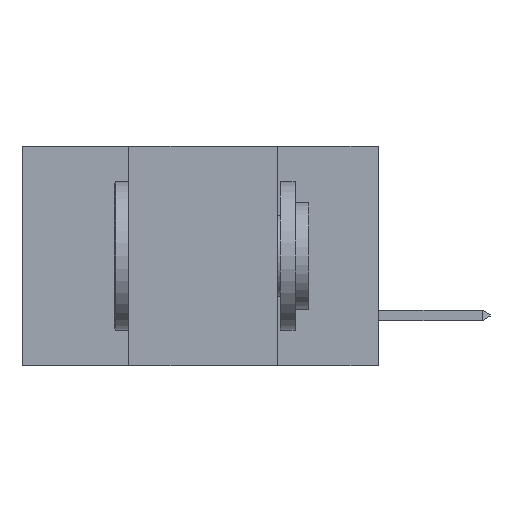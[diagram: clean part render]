
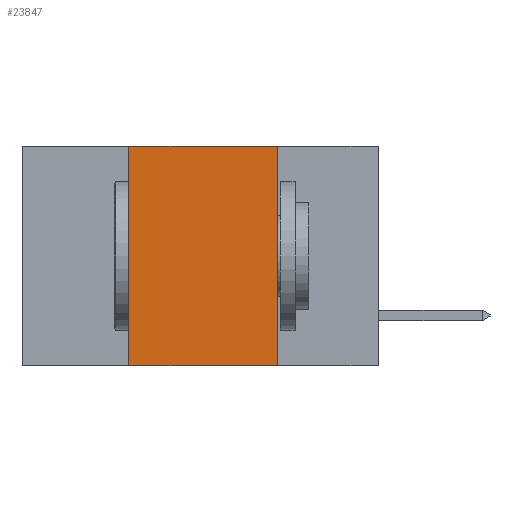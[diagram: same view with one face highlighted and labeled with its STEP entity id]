
A CAD part, left-side view. The second image highlights one B-rep face of the part: STEP entity #23847.
In plain terms, the highlighted planar face has unit normal (-1, 0, 0).
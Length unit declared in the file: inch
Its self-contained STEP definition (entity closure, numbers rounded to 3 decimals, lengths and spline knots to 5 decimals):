
#33 = VECTOR ( 'NONE', #9868, 39.37008 ) ;
#68 = LINE ( 'NONE', #454, #15232 ) ;
#454 = CARTESIAN_POINT ( 'NONE',  ( 0., 0.42, 0. ) ) ;
#1614 = CARTESIAN_POINT ( 'NONE',  ( 0., 0.42, 0. ) ) ;
#2110 = EDGE_CURVE ( 'NONE', #12741, #16547, #10633, .T. ) ;
#2787 = EDGE_CURVE ( 'NONE', #6114, #9999, #25137, .T. ) ;
#3353 = CARTESIAN_POINT ( 'NONE',  ( 0., 0.6, -0.37 ) ) ;
#3735 = ORIENTED_EDGE ( 'NONE', *, *, #16699, .F. ) ;
#4268 = CARTESIAN_POINT ( 'NONE',  ( 0., 0.17, -0.37 ) ) ;
#5247 = EDGE_LOOP ( 'NONE', ( #3735, #24932, #14243, #9458 ) ) ;
#5860 = PLANE ( 'NONE',  #14925 ) ;
#6114 = VERTEX_POINT ( 'NONE', #1614 ) ;
#9458 = ORIENTED_EDGE ( 'NONE', *, *, #2110, .T. ) ;
#9756 = DIRECTION ( 'NONE',  ( 0., 0., -1. ) ) ;
#9868 = DIRECTION ( 'NONE',  ( 0., -1., 0. ) ) ;
#9999 = VERTEX_POINT ( 'NONE', #10350 ) ;
#10350 = CARTESIAN_POINT ( 'NONE',  ( 0., 0.17, 0. ) ) ;
#10398 = DIRECTION ( 'NONE',  ( 0., 0., 1. ) ) ;
#10633 = LINE ( 'NONE', #3353, #33 ) ;
#11155 = CARTESIAN_POINT ( 'NONE',  ( 0., 0.6, 0. ) ) ;
#12680 = CARTESIAN_POINT ( 'NONE',  ( 0., 0.42, -0.37 ) ) ;
#12741 = VERTEX_POINT ( 'NONE', #12680 ) ;
#14243 = ORIENTED_EDGE ( 'NONE', *, *, #17294, .F. ) ;
#14925 = AXIS2_PLACEMENT_3D ( 'NONE', #19468, #21389, #9756 ) ;
#15232 = VECTOR ( 'NONE', #10398, 39.37008 ) ;
#16401 = DIRECTION ( 'NONE',  ( 0., 0., -1. ) ) ;
#16479 = CARTESIAN_POINT ( 'NONE',  ( 0., 0.17, 0. ) ) ;
#16547 = VERTEX_POINT ( 'NONE', #4268 ) ;
#16699 = EDGE_CURVE ( 'NONE', #9999, #16547, #24659, .T. ) ;
#17294 = EDGE_CURVE ( 'NONE', #12741, #6114, #68, .T. ) ;
#18802 = FACE_OUTER_BOUND ( 'NONE', #5247, .T. ) ;
#19468 = CARTESIAN_POINT ( 'NONE',  ( 0., 0.6, 0. ) ) ;
#19541 = DIRECTION ( 'NONE',  ( 0., -1., 0. ) ) ;
#20125 = VECTOR ( 'NONE', #16401, 39.37008 ) ;
#21230 = VECTOR ( 'NONE', #19541, 39.37008 ) ;
#21389 = DIRECTION ( 'NONE',  ( 1., 0., 0. ) ) ;
#23847 = ADVANCED_FACE ( 'NONE', ( #18802 ), #5860, .F. ) ;
#24659 = LINE ( 'NONE', #16479, #20125 ) ;
#24932 = ORIENTED_EDGE ( 'NONE', *, *, #2787, .F. ) ;
#25137 = LINE ( 'NONE', #11155, #21230 ) ;
